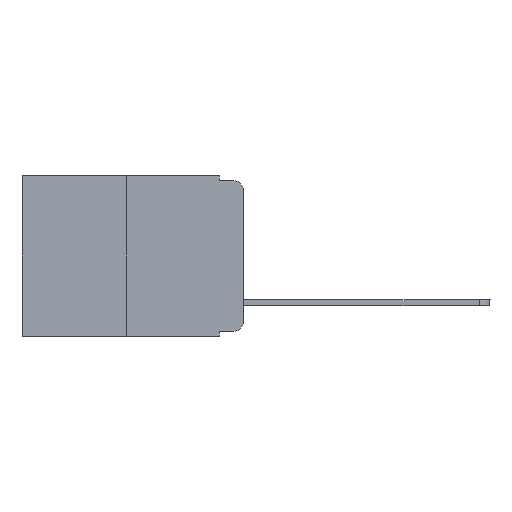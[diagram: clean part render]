
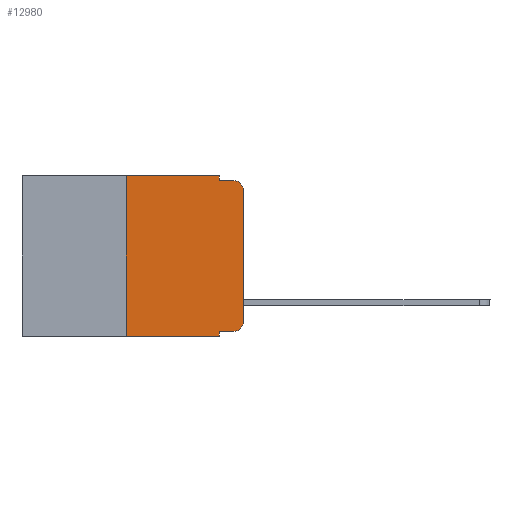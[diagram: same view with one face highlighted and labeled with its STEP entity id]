
A CAD part, left-side view. The second image highlights one B-rep face of the part: STEP entity #12980.
In plain terms, the highlighted planar face has unit normal (-1, 0, 0).
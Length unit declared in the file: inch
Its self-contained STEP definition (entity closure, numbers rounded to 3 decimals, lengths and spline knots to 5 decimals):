
#201 = VERTEX_POINT ( 'NONE', #3723 ) ;
#803 = LINE ( 'NONE', #4426, #10513 ) ;
#956 = CARTESIAN_POINT ( 'NONE',  ( 0., 0.051, 0. ) ) ;
#971 = DIRECTION ( 'NONE',  ( 0., -1., 0. ) ) ;
#1078 = ORIENTED_EDGE ( 'NONE', *, *, #6491, .T. ) ;
#1364 = ORIENTED_EDGE ( 'NONE', *, *, #12703, .F. ) ;
#1403 = ORIENTED_EDGE ( 'NONE', *, *, #1993, .F. ) ;
#1441 = DIRECTION ( 'NONE',  ( 0., 0., -1. ) ) ;
#1462 = ORIENTED_EDGE ( 'NONE', *, *, #5194, .T. ) ;
#1993 = EDGE_CURVE ( 'NONE', #9544, #3538, #9520, .T. ) ;
#2314 = VERTEX_POINT ( 'NONE', #3982 ) ;
#2356 = FACE_OUTER_BOUND ( 'NONE', #8308, .T. ) ;
#2402 = DIRECTION ( 'NONE',  ( 0., 0., -1. ) ) ;
#2442 = VECTOR ( 'NONE', #3828, 39.37008 ) ;
#2651 = CARTESIAN_POINT ( 'NONE',  ( 0., 0.02, -0.03 ) ) ;
#3067 = EDGE_CURVE ( 'NONE', #9544, #2314, #7099, .T. ) ;
#3212 = EDGE_CURVE ( 'NONE', #4352, #3538, #9668, .T. ) ;
#3253 = ORIENTED_EDGE ( 'NONE', *, *, #6655, .T. ) ;
#3470 = CARTESIAN_POINT ( 'NONE',  ( 0., 0.02, -0.313 ) ) ;
#3475 = CARTESIAN_POINT ( 'NONE',  ( 0., 0.051, -0.333 ) ) ;
#3538 = VERTEX_POINT ( 'NONE', #8699 ) ;
#3546 = VECTOR ( 'NONE', #11034, 39.37008 ) ;
#3723 = CARTESIAN_POINT ( 'NONE',  ( 0., 0.25, 0. ) ) ;
#3725 = CARTESIAN_POINT ( 'NONE',  ( 0., 0.051, 0. ) ) ;
#3796 = CARTESIAN_POINT ( 'NONE',  ( 0., 0.051, 0. ) ) ;
#3828 = DIRECTION ( 'NONE',  ( 0., 0., -1. ) ) ;
#3833 = DIRECTION ( 'NONE',  ( 1., 0., 0. ) ) ;
#3982 = CARTESIAN_POINT ( 'NONE',  ( 0., 0.02, -0.333 ) ) ;
#4254 = DIRECTION ( 'NONE',  ( 0., -1., 0. ) ) ;
#4352 = VERTEX_POINT ( 'NONE', #10735 ) ;
#4426 = CARTESIAN_POINT ( 'NONE',  ( 0., 0., 0. ) ) ;
#4476 = DIRECTION ( 'NONE',  ( 0., 0., 1. ) ) ;
#4852 = AXIS2_PLACEMENT_3D ( 'NONE', #7346, #3833, #1441 ) ;
#4964 = VECTOR ( 'NONE', #5936, 39.37008 ) ;
#5194 = EDGE_CURVE ( 'NONE', #6195, #14506, #5701, .T. ) ;
#5500 = AXIS2_PLACEMENT_3D ( 'NONE', #2651, #6360, #2402 ) ;
#5701 = CIRCLE ( 'NONE', #5500, 0.02 ) ;
#5802 = CARTESIAN_POINT ( 'NONE',  ( 0., 0.473, 0. ) ) ;
#5936 = DIRECTION ( 'NONE',  ( 0., -1., 0. ) ) ;
#6106 = LINE ( 'NONE', #3796, #12440 ) ;
#6195 = VERTEX_POINT ( 'NONE', #8432 ) ;
#6360 = DIRECTION ( 'NONE',  ( -1., 0., 0. ) ) ;
#6411 = CARTESIAN_POINT ( 'NONE',  ( 0., 0.051, -0.333 ) ) ;
#6491 = EDGE_CURVE ( 'NONE', #8413, #6195, #803, .T. ) ;
#6655 = EDGE_CURVE ( 'NONE', #2314, #8413, #13667, .T. ) ;
#6682 = LINE ( 'NONE', #5802, #8708 ) ;
#6892 = VECTOR ( 'NONE', #8808, 39.37008 ) ;
#7099 = LINE ( 'NONE', #6411, #6892 ) ;
#7225 = ORIENTED_EDGE ( 'NONE', *, *, #10256, .F. ) ;
#7346 = CARTESIAN_POINT ( 'NONE',  ( 0., 0.473, 0. ) ) ;
#7499 = VERTEX_POINT ( 'NONE', #956 ) ;
#7500 = PLANE ( 'NONE',  #4852 ) ;
#7863 = VECTOR ( 'NONE', #4254, 39.37008 ) ;
#8171 = LINE ( 'NONE', #9632, #4964 ) ;
#8201 = ORIENTED_EDGE ( 'NONE', *, *, #3212, .T. ) ;
#8308 = EDGE_LOOP ( 'NONE', ( #1078, #1462, #7225, #12030, #1364, #14823, #8201, #1403, #9163, #3253 ) ) ;
#8413 = VERTEX_POINT ( 'NONE', #14453 ) ;
#8432 = CARTESIAN_POINT ( 'NONE',  ( 0., 0., -0.03 ) ) ;
#8699 = CARTESIAN_POINT ( 'NONE',  ( 0., 0.051, -0.343 ) ) ;
#8708 = VECTOR ( 'NONE', #971, 39.37008 ) ;
#8808 = DIRECTION ( 'NONE',  ( 0., -1., 0. ) ) ;
#9038 = EDGE_CURVE ( 'NONE', #7499, #10538, #6106, .T. ) ;
#9163 = ORIENTED_EDGE ( 'NONE', *, *, #3067, .T. ) ;
#9490 = DIRECTION ( 'NONE',  ( -1., 0., 0. ) ) ;
#9520 = LINE ( 'NONE', #3725, #2442 ) ;
#9544 = VERTEX_POINT ( 'NONE', #3475 ) ;
#9632 = CARTESIAN_POINT ( 'NONE',  ( 0., 0.051, -0.01 ) ) ;
#9668 = LINE ( 'NONE', #10324, #7863 ) ;
#9778 = CARTESIAN_POINT ( 'NONE',  ( 0., 0.25, 0. ) ) ;
#10256 = EDGE_CURVE ( 'NONE', #10538, #14506, #8171, .T. ) ;
#10324 = CARTESIAN_POINT ( 'NONE',  ( 0., 0.473, -0.343 ) ) ;
#10513 = VECTOR ( 'NONE', #4476, 39.37008 ) ;
#10538 = VERTEX_POINT ( 'NONE', #13484 ) ;
#10735 = CARTESIAN_POINT ( 'NONE',  ( 0., 0.25, -0.343 ) ) ;
#11034 = DIRECTION ( 'NONE',  ( 0., 0., 1. ) ) ;
#11894 = AXIS2_PLACEMENT_3D ( 'NONE', #3470, #9490, #14115 ) ;
#12030 = ORIENTED_EDGE ( 'NONE', *, *, #9038, .F. ) ;
#12154 = DIRECTION ( 'NONE',  ( 0., 0., -1. ) ) ;
#12308 = EDGE_CURVE ( 'NONE', #4352, #201, #14743, .T. ) ;
#12440 = VECTOR ( 'NONE', #12154, 39.37008 ) ;
#12703 = EDGE_CURVE ( 'NONE', #201, #7499, #6682, .T. ) ;
#12980 = ADVANCED_FACE ( 'NONE', ( #2356 ), #7500, .F. ) ;
#13484 = CARTESIAN_POINT ( 'NONE',  ( 0., 0.051, -0.01 ) ) ;
#13593 = CARTESIAN_POINT ( 'NONE',  ( 0., 0.02, -0.01 ) ) ;
#13667 = CIRCLE ( 'NONE', #11894, 0.02 ) ;
#14115 = DIRECTION ( 'NONE',  ( 0., 0., -1. ) ) ;
#14453 = CARTESIAN_POINT ( 'NONE',  ( 0., 0., -0.313 ) ) ;
#14506 = VERTEX_POINT ( 'NONE', #13593 ) ;
#14743 = LINE ( 'NONE', #9778, #3546 ) ;
#14823 = ORIENTED_EDGE ( 'NONE', *, *, #12308, .F. ) ;
